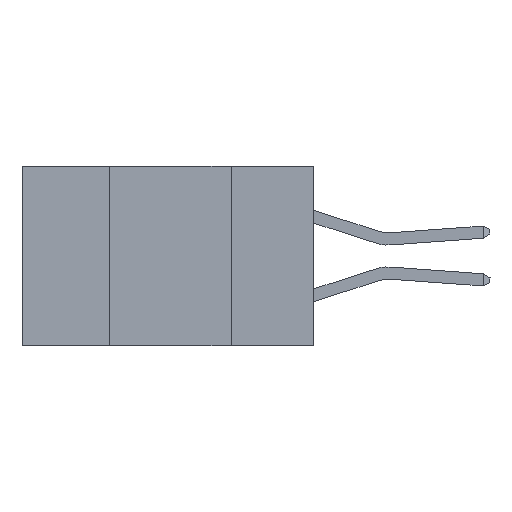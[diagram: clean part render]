
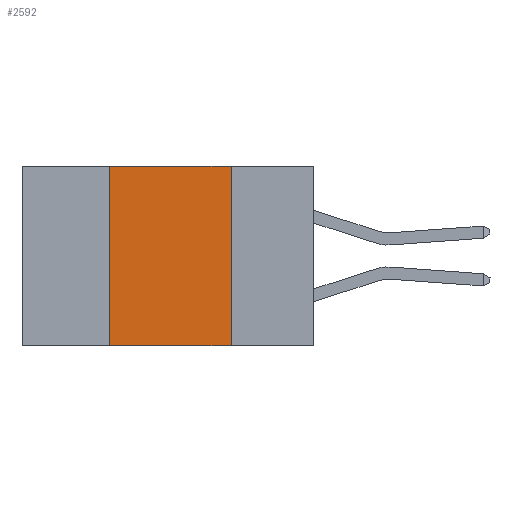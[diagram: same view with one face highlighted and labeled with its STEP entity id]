
A CAD part, left-side view. The second image highlights one B-rep face of the part: STEP entity #2592.
In plain terms, the highlighted planar face has unit normal (-1, 0, 0).
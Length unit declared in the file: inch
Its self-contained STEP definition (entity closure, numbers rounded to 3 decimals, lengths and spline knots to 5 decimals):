
#131 = PLANE ( 'NONE',  #12128 ) ;
#1111 = VECTOR ( 'NONE', #13543, 39.37008 ) ;
#2388 = EDGE_CURVE ( 'NONE', #24791, #20191, #23857, .T. ) ;
#2592 = ADVANCED_FACE ( 'NONE', ( #6702 ), #131, .F. ) ;
#2647 = DIRECTION ( 'NONE',  ( 0., 0., -1. ) ) ;
#3837 = DIRECTION ( 'NONE',  ( 0., -1., 0. ) ) ;
#4520 = VECTOR ( 'NONE', #3837, 39.37008 ) ;
#6233 = VECTOR ( 'NONE', #2647, 39.37008 ) ;
#6270 = ORIENTED_EDGE ( 'NONE', *, *, #2388, .F. ) ;
#6445 = VERTEX_POINT ( 'NONE', #17117 ) ;
#6458 = LINE ( 'NONE', #11730, #1111 ) ;
#6544 = ORIENTED_EDGE ( 'NONE', *, *, #20217, .T. ) ;
#6702 = FACE_OUTER_BOUND ( 'NONE', #22292, .T. ) ;
#7156 = ORIENTED_EDGE ( 'NONE', *, *, #14068, .F. ) ;
#7348 = LINE ( 'NONE', #15779, #4520 ) ;
#8229 = CARTESIAN_POINT ( 'NONE',  ( 0., 0.6, 0. ) ) ;
#8566 = VECTOR ( 'NONE', #13480, 39.37008 ) ;
#11190 = LINE ( 'NONE', #18523, #6233 ) ;
#11730 = CARTESIAN_POINT ( 'NONE',  ( 0., 0.6, -0.37 ) ) ;
#12128 = AXIS2_PLACEMENT_3D ( 'NONE', #8229, #14109, #17863 ) ;
#12891 = CARTESIAN_POINT ( 'NONE',  ( 0., 0.42, -0.37 ) ) ;
#13480 = DIRECTION ( 'NONE',  ( 0., 0., 1. ) ) ;
#13543 = DIRECTION ( 'NONE',  ( 0., -1., 0. ) ) ;
#13583 = ORIENTED_EDGE ( 'NONE', *, *, #21157, .F. ) ;
#14068 = EDGE_CURVE ( 'NONE', #6445, #24251, #11190, .T. ) ;
#14109 = DIRECTION ( 'NONE',  ( 1., 0., 0. ) ) ;
#15779 = CARTESIAN_POINT ( 'NONE',  ( 0., 0.6, 0. ) ) ;
#16906 = CARTESIAN_POINT ( 'NONE',  ( 0., 0.42, 0. ) ) ;
#17117 = CARTESIAN_POINT ( 'NONE',  ( 0., 0.17, 0. ) ) ;
#17863 = DIRECTION ( 'NONE',  ( 0., 0., -1. ) ) ;
#18523 = CARTESIAN_POINT ( 'NONE',  ( 0., 0.17, 0. ) ) ;
#19035 = CARTESIAN_POINT ( 'NONE',  ( 0., 0.17, -0.37 ) ) ;
#20191 = VERTEX_POINT ( 'NONE', #25895 ) ;
#20217 = EDGE_CURVE ( 'NONE', #24791, #24251, #6458, .T. ) ;
#21157 = EDGE_CURVE ( 'NONE', #20191, #6445, #7348, .T. ) ;
#22292 = EDGE_LOOP ( 'NONE', ( #7156, #13583, #6270, #6544 ) ) ;
#23857 = LINE ( 'NONE', #16906, #8566 ) ;
#24251 = VERTEX_POINT ( 'NONE', #19035 ) ;
#24791 = VERTEX_POINT ( 'NONE', #12891 ) ;
#25895 = CARTESIAN_POINT ( 'NONE',  ( 0., 0.42, 0. ) ) ;
